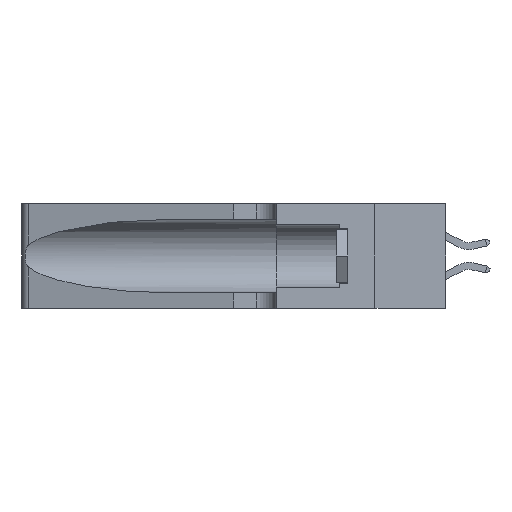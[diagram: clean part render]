
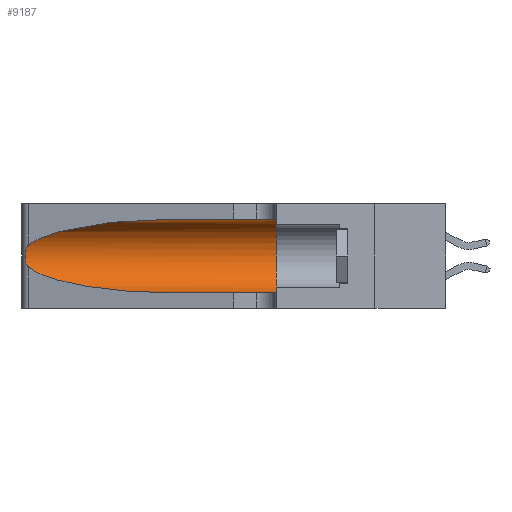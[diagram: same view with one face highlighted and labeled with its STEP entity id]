
A CAD part, left-side view. The second image highlights one B-rep face of the part: STEP entity #9187.
In plain terms, the highlighted cylindrical face has radius 3.308 mm (diameter 6.617 mm), a partial arc.
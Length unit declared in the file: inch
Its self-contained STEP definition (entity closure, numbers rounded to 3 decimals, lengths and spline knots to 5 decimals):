
#313 = CARTESIAN_POINT ( 'NONE',  ( 0.26017, 1.23833, 0.17102 ) ) ;
#915 = CARTESIAN_POINT ( 'NONE',  ( 0.1305, 0.35, 0.185 ) ) ;
#974 = DIRECTION ( 'NONE',  ( 0., -1., 0. ) ) ;
#3494 = EDGE_CURVE ( 'NONE', #6756, #29830, #16374, .T. ) ;
#4746 = AXIS2_PLACEMENT_3D ( 'NONE', #16868, #14418, #14327 ) ;
#4752 = VERTEX_POINT ( 'NONE', #18609 ) ;
#5130 = CARTESIAN_POINT ( 'NONE',  ( 0.26075, 1.23896, 0.178 ) ) ;
#6171 = CIRCLE ( 'NONE', #17856, 0.13025 ) ;
#6423 =( BOUNDED_CURVE ( )  B_SPLINE_CURVE ( 3, ( #31261, #16681, #22321, #26498 ),
 .UNSPECIFIED., .F., .T. ) 
 B_SPLINE_CURVE_WITH_KNOTS ( ( 4, 4 ),
 ( 3.44316, 4.71239 ),
 .UNSPECIFIED. ) 
 CURVE ( )  GEOMETRIC_REPRESENTATION_ITEM ( )  RATIONAL_B_SPLINE_CURVE ( ( 1., 0.87, 0.87, 1. ) ) 
 REPRESENTATION_ITEM ( '' )  );
#6502 = CARTESIAN_POINT ( 'NONE',  ( 0.25487, 1.22718, 0.22369 ) ) ;
#6721 = DIRECTION ( 'NONE',  ( 0., -1., 0. ) ) ;
#6756 = VERTEX_POINT ( 'NONE', #11712 ) ;
#6777 = CARTESIAN_POINT ( 'NONE',  ( 0.25787, 1.23484, 0.2124 ) ) ;
#7451 = LINE ( 'NONE', #15123, #13164 ) ;
#7889 = CARTESIAN_POINT ( 'NONE',  ( 0.25487, 1.22718, 0.22369 ) ) ;
#8548 = DIRECTION ( 'NONE',  ( 0., 0., 1. ) ) ;
#9187 = ADVANCED_FACE ( 'NONE', ( #17427 ), #24280, .F. ) ;
#9309 = CARTESIAN_POINT ( 'NONE',  ( 0.26018, 1.23835, 0.19895 ) ) ;
#10549 = DIRECTION ( 'NONE',  ( 0., 1., 0. ) ) ;
#10756 = ORIENTED_EDGE ( 'NONE', *, *, #3494, .F. ) ;
#11072 = VECTOR ( 'NONE', #6721, 39.37008 ) ;
#11204 = VERTEX_POINT ( 'NONE', #12395 ) ;
#11712 = CARTESIAN_POINT ( 'NONE',  ( 0.1305, 0.72297, 0.31525 ) ) ;
#12395 = CARTESIAN_POINT ( 'NONE',  ( 0.1305, 0.35, 0.05475 ) ) ;
#13164 = VECTOR ( 'NONE', #974, 39.37008 ) ;
#13208 = EDGE_CURVE ( 'NONE', #4752, #11204, #7451, .T. ) ;
#13656 = CARTESIAN_POINT ( 'NONE',  ( 0.25487, 1.22718, 0.14631 ) ) ;
#14327 = DIRECTION ( 'NONE',  ( 0., 0., -1. ) ) ;
#14418 = DIRECTION ( 'NONE',  ( 0., -1., 0. ) ) ;
#15038 = EDGE_CURVE ( 'NONE', #6756, #15773, #23355, .T. ) ;
#15123 = CARTESIAN_POINT ( 'NONE',  ( 0.1305, 1.61858, 0.05475 ) ) ;
#15172 = CARTESIAN_POINT ( 'NONE',  ( 0.25639, 1.23186, 0.15144 ) ) ;
#15439 = ORIENTED_EDGE ( 'NONE', *, *, #15038, .T. ) ;
#15773 = VERTEX_POINT ( 'NONE', #6502 ) ;
#16374 = LINE ( 'NONE', #19033, #11072 ) ;
#16681 = CARTESIAN_POINT ( 'NONE',  ( 0.2373, 1.15595, 0.08982 ) ) ;
#16700 = CARTESIAN_POINT ( 'NONE',  ( 0.25854, 1.2359, 0.20912 ) ) ;
#16868 = CARTESIAN_POINT ( 'NONE',  ( 0.1305, 1.61858, 0.185 ) ) ;
#17117 = CARTESIAN_POINT ( 'NONE',  ( 0.26075, 1.23896, 0.19203 ) ) ;
#17311 = CARTESIAN_POINT ( 'NONE',  ( 0.25856, 1.23593, 0.16098 ) ) ;
#17371 = ORIENTED_EDGE ( 'NONE', *, *, #19398, .T. ) ;
#17427 = FACE_OUTER_BOUND ( 'NONE', #23038, .T. ) ;
#17676 = CARTESIAN_POINT ( 'NONE',  ( 0.25555, 1.22994, 0.2215 ) ) ;
#17856 = AXIS2_PLACEMENT_3D ( 'NONE', #915, #10549, #8548 ) ;
#18609 = CARTESIAN_POINT ( 'NONE',  ( 0.1305, 0.72297, 0.05475 ) ) ;
#18641 = CARTESIAN_POINT ( 'NONE',  ( 0.1305, 0.35, 0.31525 ) ) ;
#19033 = CARTESIAN_POINT ( 'NONE',  ( 0.1305, 1.61858, 0.31525 ) ) ;
#19384 = CARTESIAN_POINT ( 'NONE',  ( 0.1305, 0.72297, 0.31525 ) ) ;
#19398 = EDGE_CURVE ( 'NONE', #28811, #4752, #6423, .T. ) ;
#20778 = CARTESIAN_POINT ( 'NONE',  ( 0.25555, 1.22993, 0.14849 ) ) ;
#21339 = ORIENTED_EDGE ( 'NONE', *, *, #22348, .T. ) ;
#21720 = CARTESIAN_POINT ( 'NONE',  ( 0.25789, 1.23486, 0.15765 ) ) ;
#21798 = CARTESIAN_POINT ( 'NONE',  ( 0.18966, 0.96281, 0.31525 ) ) ;
#22321 = CARTESIAN_POINT ( 'NONE',  ( 0.18966, 0.96281, 0.05475 ) ) ;
#22348 = EDGE_CURVE ( 'NONE', #15773, #28811, #27631, .T. ) ;
#23038 = EDGE_LOOP ( 'NONE', ( #15439, #21339, #17371, #23668, #23272, #10756 ) ) ;
#23272 = ORIENTED_EDGE ( 'NONE', *, *, #24967, .F. ) ;
#23355 =( BOUNDED_CURVE ( )  B_SPLINE_CURVE ( 3, ( #19384, #21798, #24138, #26400 ),
 .UNSPECIFIED., .F., .T. ) 
 B_SPLINE_CURVE_WITH_KNOTS ( ( 4, 4 ),
 ( 1.5708, 2.84003 ),
 .UNSPECIFIED. ) 
 CURVE ( )  GEOMETRIC_REPRESENTATION_ITEM ( )  RATIONAL_B_SPLINE_CURVE ( ( 1., 0.87, 0.87, 1. ) ) 
 REPRESENTATION_ITEM ( '' )  );
#23668 = ORIENTED_EDGE ( 'NONE', *, *, #13208, .T. ) ;
#24138 = CARTESIAN_POINT ( 'NONE',  ( 0.2373, 1.15595, 0.28018 ) ) ;
#24280 = CYLINDRICAL_SURFACE ( 'NONE', #4746, 0.13025 ) ;
#24967 = EDGE_CURVE ( 'NONE', #29830, #11204, #6171, .T. ) ;
#26400 = CARTESIAN_POINT ( 'NONE',  ( 0.25487, 1.22718, 0.22369 ) ) ;
#26498 = CARTESIAN_POINT ( 'NONE',  ( 0.1305, 0.72297, 0.05475 ) ) ;
#27631 = B_SPLINE_CURVE_WITH_KNOTS ( 'NONE', 3,
 ( #7889, #17676, #30970, #6777, #16700, #9309, #17117, #5130, #313, #17311, #21720, #15172, #20778, #30070 ),
 .UNSPECIFIED., .F., .F.,
 ( 4, 2, 2, 2, 2, 2, 4 ),
 ( 0., 0.00027, 0.00053, 0.00107, 0.0016, 0.00187, 0.00214 ),
 .UNSPECIFIED. ) ;
#28811 = VERTEX_POINT ( 'NONE', #13656 ) ;
#29830 = VERTEX_POINT ( 'NONE', #18641 ) ;
#30070 = CARTESIAN_POINT ( 'NONE',  ( 0.25487, 1.22718, 0.14631 ) ) ;
#30970 = CARTESIAN_POINT ( 'NONE',  ( 0.25639, 1.23184, 0.21858 ) ) ;
#31261 = CARTESIAN_POINT ( 'NONE',  ( 0.25487, 1.22718, 0.14631 ) ) ;
